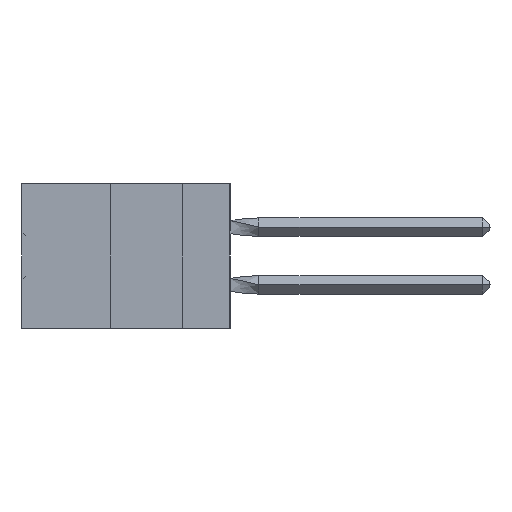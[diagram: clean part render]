
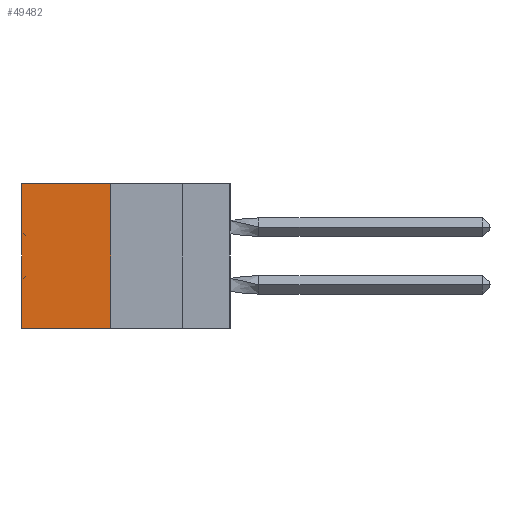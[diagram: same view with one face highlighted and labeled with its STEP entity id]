
A CAD part, left-side view. The second image highlights one B-rep face of the part: STEP entity #49482.
In plain terms, the highlighted planar face has unit normal (-1, 0, 0).
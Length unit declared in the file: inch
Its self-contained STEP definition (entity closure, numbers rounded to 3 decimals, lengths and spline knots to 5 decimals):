
#81 = ORIENTED_EDGE ( 'NONE', *, *, #40382, .F. ) ;
#1260 = LINE ( 'NONE', #33825, #24178 ) ;
#3489 = VECTOR ( 'NONE', #37158, 39.37008 ) ;
#3930 = ORIENTED_EDGE ( 'NONE', *, *, #53174, .T. ) ;
#5009 = LINE ( 'NONE', #5913, #48700 ) ;
#5774 = DIRECTION ( 'NONE',  ( 0., 0., -1. ) ) ;
#5913 = CARTESIAN_POINT ( 'NONE',  ( 0.305, 0.72, -0.5 ) ) ;
#7188 = AXIS2_PLACEMENT_3D ( 'NONE', #20950, #31342, #35184 ) ;
#10768 = DIRECTION ( 'NONE',  ( 0., 1., 0. ) ) ;
#15484 = VECTOR ( 'NONE', #10768, 39.37008 ) ;
#16336 = ORIENTED_EDGE ( 'NONE', *, *, #19515, .F. ) ;
#19389 = VERTEX_POINT ( 'NONE', #42844 ) ;
#19515 = EDGE_CURVE ( 'NONE', #45342, #19389, #27858, .T. ) ;
#20950 = CARTESIAN_POINT ( 'NONE',  ( 0.305, 0.413, -0.5 ) ) ;
#24178 = VECTOR ( 'NONE', #5774, 39.37008 ) ;
#27724 = EDGE_CURVE ( 'NONE', #44872, #36755, #46351, .T. ) ;
#27858 = LINE ( 'NONE', #50720, #3489 ) ;
#30666 = EDGE_LOOP ( 'NONE', ( #3930, #16336, #81, #45497 ) ) ;
#31342 = DIRECTION ( 'NONE',  ( 1., 0., 0. ) ) ;
#32398 = CARTESIAN_POINT ( 'NONE',  ( 0.305, 0.413, 0. ) ) ;
#33825 = CARTESIAN_POINT ( 'NONE',  ( 0.305, 0.413, -0.5 ) ) ;
#35184 = DIRECTION ( 'NONE',  ( 0., 0., -1. ) ) ;
#36755 = VERTEX_POINT ( 'NONE', #46954 ) ;
#37158 = DIRECTION ( 'NONE',  ( 0., 1., 0. ) ) ;
#40382 = EDGE_CURVE ( 'NONE', #44872, #45342, #1260, .T. ) ;
#40628 = CARTESIAN_POINT ( 'NONE',  ( 0.305, 0.413, 0. ) ) ;
#40687 = FACE_OUTER_BOUND ( 'NONE', #30666, .T. ) ;
#42844 = CARTESIAN_POINT ( 'NONE',  ( 0.305, 0.72, -0.5 ) ) ;
#44872 = VERTEX_POINT ( 'NONE', #40628 ) ;
#45342 = VERTEX_POINT ( 'NONE', #52199 ) ;
#45497 = ORIENTED_EDGE ( 'NONE', *, *, #27724, .T. ) ;
#46351 = LINE ( 'NONE', #32398, #15484 ) ;
#46584 = DIRECTION ( 'NONE',  ( 0., 0., -1. ) ) ;
#46954 = CARTESIAN_POINT ( 'NONE',  ( 0.305, 0.72, 0. ) ) ;
#48394 = PLANE ( 'NONE',  #7188 ) ;
#48700 = VECTOR ( 'NONE', #46584, 39.37008 ) ;
#49482 = ADVANCED_FACE ( 'NONE', ( #40687 ), #48394, .F. ) ;
#50720 = CARTESIAN_POINT ( 'NONE',  ( 0.305, 0.413, -0.5 ) ) ;
#52199 = CARTESIAN_POINT ( 'NONE',  ( 0.305, 0.413, -0.5 ) ) ;
#53174 = EDGE_CURVE ( 'NONE', #36755, #19389, #5009, .T. ) ;
